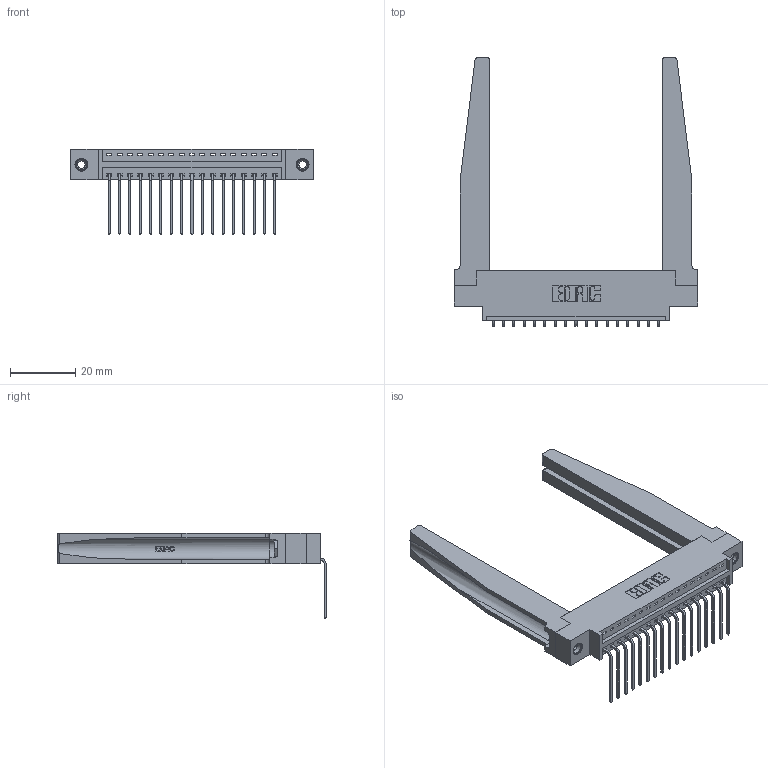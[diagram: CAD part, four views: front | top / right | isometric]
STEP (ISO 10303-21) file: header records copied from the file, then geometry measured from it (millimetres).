
FILE_DESCRIPTION (( 'STEP AP203' ), '1' );
FILE_NAME ('346-017-559-678.STEP', '2022-05-05T13:37:29', ( '' ), ( '' ), 'SwSTEP 2.0', 'SolidWorks 2020', '' );
FILE_SCHEMA (( 'CONFIG_CONTROL_DESIGN' ));
Length unit declared in the file: inch
Products named in the file (5): 345-250-001_345-250-001-102; 345-292-001_558 559 Tail - 1; 346-017-559-678; 346-220-078_345-220-078; 346 Part_0.170 Offset - 0.156 Dia-TH
Assembly tree (22 placements, depth 2):
  346-017-559-678
    346 Part_0.170 Offset - 0.156 Dia-TH
    345-292-001_558 559 Tail - 1  x17
    346-220-078_345-220-078  x2
    345-250-001_345-250-001-102  x2
Bounding box: 74.55 x 82.36 x 26.16 mm (x, y, z)
Volume: 13756.5 mm3; surface area: 15359.6 mm2
Topology: 22 solids, 22 shells, 1394 faces, 4079 edges, 2686 vertices
Faces by surface type: plane 950, cylinder 392, bspline 36, cone 12, torus 4
Entity records: 19296 total; most frequent: CARTESIAN_POINT 4232, ORIENTED_EDGE 3070, DIRECTION 2747, EDGE_CURVE 1535, VECTOR 1241, LINE 1241, VERTEX_POINT 1016, AXIS2_PLACEMENT_3D 753
